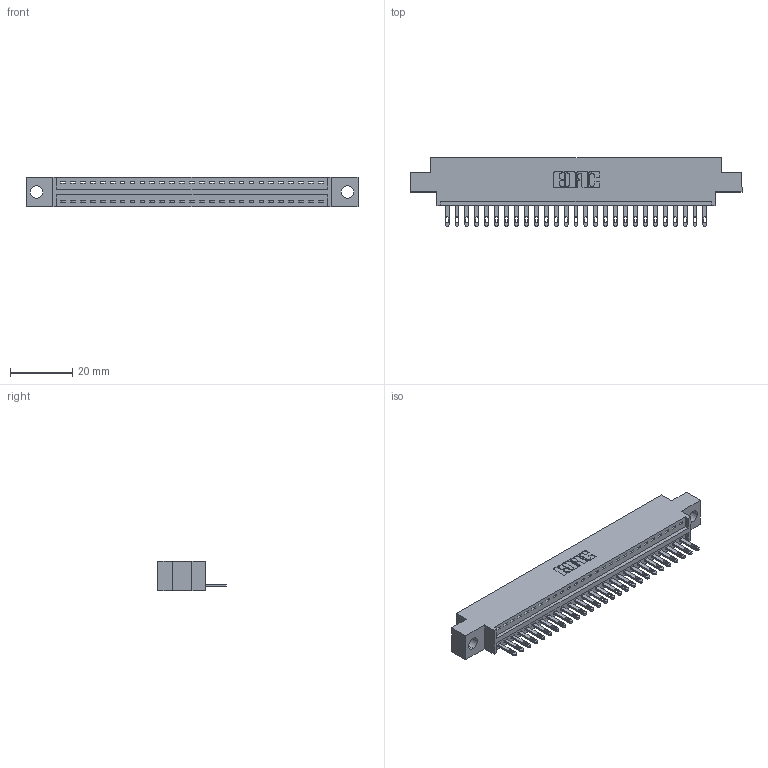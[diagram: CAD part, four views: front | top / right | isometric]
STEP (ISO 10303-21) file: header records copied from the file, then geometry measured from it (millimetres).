
FILE_DESCRIPTION (( 'STEP AP203' ), '1' );
FILE_NAME ('346-027-500-604.STEP', '2022-05-06T03:54:01', ( '' ), ( '' ), 'SwSTEP 2.0', 'SolidWorks 2020', '' );
FILE_SCHEMA (( 'CONFIG_CONTROL_DESIGN' ));
Length unit declared in the file: inch
Products named in the file (3): 346 Part_0.170 Offset - 0.156 Dia-TH; 345-292-001_345-293-100; 346-027-500-604
Assembly tree (28 placements, depth 2):
  346-027-500-604
    346 Part_0.170 Offset - 0.156 Dia-TH
    345-292-001_345-293-100  x27
Bounding box: 106.3 x 21.84 x 9.4 mm (x, y, z)
Volume: 9828 mm3; surface area: 12182.3 mm2
Topology: 28 solids, 28 shells, 1598 faces, 4913 edges, 3274 vertices
Faces by surface type: plane 1012, cylinder 586
Entity records: 19257 total; most frequent: CARTESIAN_POINT 3315, ORIENTED_EDGE 3274, DIRECTION 2943, EDGE_CURVE 1637, VECTOR 1393, LINE 1393, VERTEX_POINT 1090, AXIS2_PLACEMENT_3D 775
